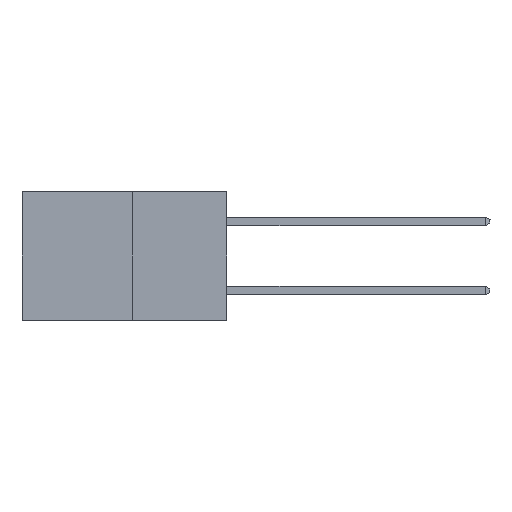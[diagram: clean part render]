
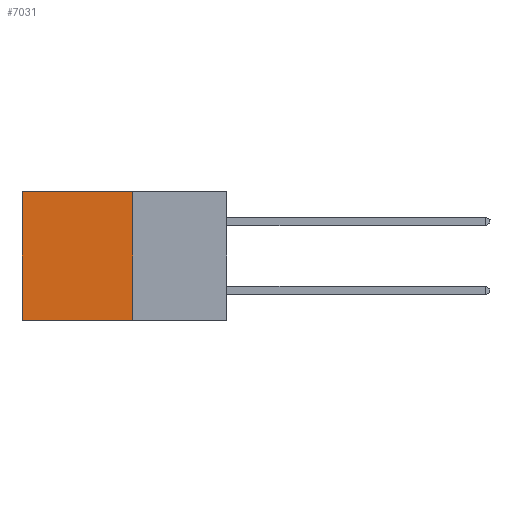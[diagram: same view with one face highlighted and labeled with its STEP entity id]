
A CAD part, left-side view. The second image highlights one B-rep face of the part: STEP entity #7031.
In plain terms, the highlighted planar face has unit normal (-1, 0, 0).
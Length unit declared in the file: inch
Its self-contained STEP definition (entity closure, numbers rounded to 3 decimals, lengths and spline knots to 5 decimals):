
#293 = EDGE_LOOP ( 'NONE', ( #3511, #5352, #9596, #10645 ) ) ;
#499 = DIRECTION ( 'NONE',  ( 0., 0., -1. ) ) ;
#1102 = CARTESIAN_POINT ( 'NONE',  ( 0.277, 0.27, 0. ) ) ;
#1306 = DIRECTION ( 'NONE',  ( 0., 1., 0. ) ) ;
#1309 = EDGE_CURVE ( 'NONE', #3354, #8245, #2434, .T. ) ;
#1318 = VERTEX_POINT ( 'NONE', #13983 ) ;
#1672 = CARTESIAN_POINT ( 'NONE',  ( 0.277, 0.27, -0.37 ) ) ;
#2077 = VECTOR ( 'NONE', #499, 39.37008 ) ;
#2167 = AXIS2_PLACEMENT_3D ( 'NONE', #13560, #10133, #3140 ) ;
#2434 = LINE ( 'NONE', #7510, #2077 ) ;
#2523 = CARTESIAN_POINT ( 'NONE',  ( 0.277, 0.27, -0.37 ) ) ;
#3091 = EDGE_CURVE ( 'NONE', #14599, #1318, #6310, .T. ) ;
#3140 = DIRECTION ( 'NONE',  ( 0., 0., -1. ) ) ;
#3354 = VERTEX_POINT ( 'NONE', #1102 ) ;
#3511 = ORIENTED_EDGE ( 'NONE', *, *, #3091, .T. ) ;
#3682 = DIRECTION ( 'NONE',  ( 0., 1., 0. ) ) ;
#3703 = VECTOR ( 'NONE', #1306, 39.37008 ) ;
#3972 = FACE_OUTER_BOUND ( 'NONE', #293, .T. ) ;
#5352 = ORIENTED_EDGE ( 'NONE', *, *, #11542, .F. ) ;
#6310 = LINE ( 'NONE', #13433, #12454 ) ;
#7031 = ADVANCED_FACE ( 'NONE', ( #3972 ), #8999, .F. ) ;
#7173 = CARTESIAN_POINT ( 'NONE',  ( 0.277, 0.27, 0. ) ) ;
#7510 = CARTESIAN_POINT ( 'NONE',  ( 0.277, 0.27, -0.37 ) ) ;
#8169 = CARTESIAN_POINT ( 'NONE',  ( 0.277, 0.59, 0. ) ) ;
#8245 = VERTEX_POINT ( 'NONE', #1672 ) ;
#8999 = PLANE ( 'NONE',  #2167 ) ;
#9430 = LINE ( 'NONE', #2523, #9790 ) ;
#9596 = ORIENTED_EDGE ( 'NONE', *, *, #1309, .F. ) ;
#9790 = VECTOR ( 'NONE', #3682, 39.37008 ) ;
#9947 = LINE ( 'NONE', #7173, #3703 ) ;
#10133 = DIRECTION ( 'NONE',  ( 1., 0., 0. ) ) ;
#10645 = ORIENTED_EDGE ( 'NONE', *, *, #12181, .T. ) ;
#11542 = EDGE_CURVE ( 'NONE', #8245, #1318, #9430, .T. ) ;
#12181 = EDGE_CURVE ( 'NONE', #3354, #14599, #9947, .T. ) ;
#12454 = VECTOR ( 'NONE', #13318, 39.37008 ) ;
#13318 = DIRECTION ( 'NONE',  ( 0., 0., -1. ) ) ;
#13433 = CARTESIAN_POINT ( 'NONE',  ( 0.277, 0.59, -0.37 ) ) ;
#13560 = CARTESIAN_POINT ( 'NONE',  ( 0.277, 0.27, -0.37 ) ) ;
#13983 = CARTESIAN_POINT ( 'NONE',  ( 0.277, 0.59, -0.37 ) ) ;
#14599 = VERTEX_POINT ( 'NONE', #8169 ) ;
